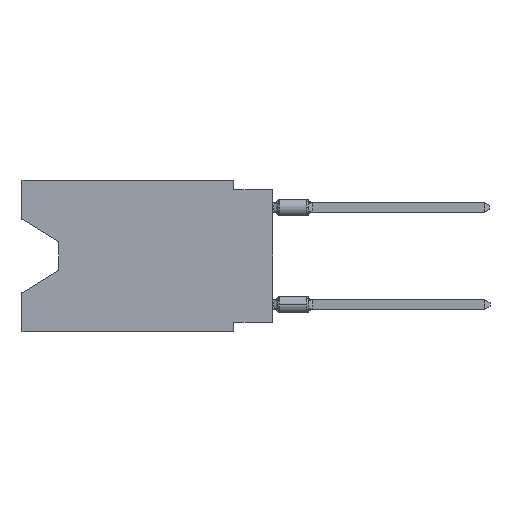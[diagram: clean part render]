
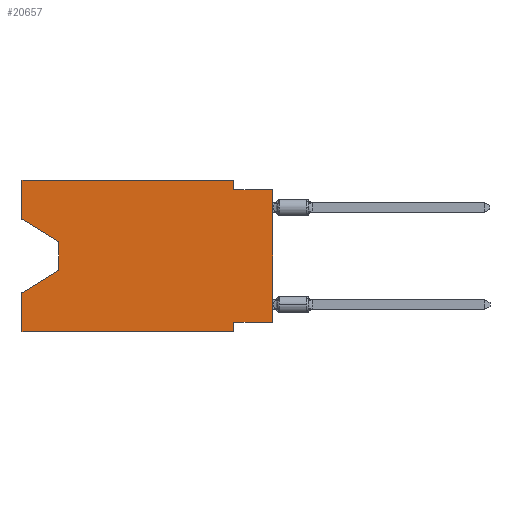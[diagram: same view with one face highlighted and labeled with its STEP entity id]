
A CAD part, left-side view. The second image highlights one B-rep face of the part: STEP entity #20657.
In plain terms, the highlighted planar face has unit normal (-1, 0, 0).
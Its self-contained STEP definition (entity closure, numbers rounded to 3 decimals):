
#172 = CARTESIAN_POINT ( 'NONE',  ( 0., 13.97, -4.013 ) ) ;
#270 = CARTESIAN_POINT ( 'NONE',  ( 0., 16.383, 0. ) ) ;
#666 = CARTESIAN_POINT ( 'NONE',  ( 0., 0., -0.635 ) ) ;
#1020 = CARTESIAN_POINT ( 'NONE',  ( 0., 13.97, -5.893 ) ) ;
#1090 = VERTEX_POINT ( 'NONE', #17927 ) ;
#1123 = ORIENTED_EDGE ( 'NONE', *, *, #8444, .T. ) ;
#1266 = VECTOR ( 'NONE', #6108, 1000. ) ;
#1345 = EDGE_CURVE ( 'NONE', #3712, #14946, #4710, .T. ) ;
#1466 = DIRECTION ( 'NONE',  ( 0., 0., 1. ) ) ;
#2115 = LINE ( 'NONE', #22886, #17380 ) ;
#2216 = PLANE ( 'NONE',  #22146 ) ;
#2451 = DIRECTION ( 'NONE',  ( 1., 0., 0. ) ) ;
#2823 = DIRECTION ( 'NONE',  ( 0., -1., 0. ) ) ;
#3032 = EDGE_CURVE ( 'NONE', #1090, #3712, #23635, .T. ) ;
#3294 = CARTESIAN_POINT ( 'NONE',  ( 0., 0., 0. ) ) ;
#3623 = VECTOR ( 'NONE', #15454, 1000. ) ;
#3646 = DIRECTION ( 'NONE',  ( 0., -1., 0. ) ) ;
#3660 = VECTOR ( 'NONE', #1466, 1000. ) ;
#3712 = VERTEX_POINT ( 'NONE', #14829 ) ;
#3999 = EDGE_CURVE ( 'NONE', #6644, #1090, #4670, .T. ) ;
#4010 = CARTESIAN_POINT ( 'NONE',  ( 0., 16.383, -2.546 ) ) ;
#4031 = CARTESIAN_POINT ( 'NONE',  ( 0., 16.383, -2.546 ) ) ;
#4294 = VERTEX_POINT ( 'NONE', #12176 ) ;
#4529 = VERTEX_POINT ( 'NONE', #20146 ) ;
#4670 = LINE ( 'NONE', #4904, #5822 ) ;
#4710 = LINE ( 'NONE', #666, #17588 ) ;
#4880 = ORIENTED_EDGE ( 'NONE', *, *, #17464, .F. ) ;
#4904 = CARTESIAN_POINT ( 'NONE',  ( 0., 16.383, 0. ) ) ;
#5822 = VECTOR ( 'NONE', #2823, 1000. ) ;
#5956 = VECTOR ( 'NONE', #19728, 1000. ) ;
#6108 = DIRECTION ( 'NONE',  ( 0., 0., -1. ) ) ;
#6146 = DIRECTION ( 'NONE',  ( 0., 0., -1. ) ) ;
#6256 = ORIENTED_EDGE ( 'NONE', *, *, #12687, .T. ) ;
#6288 = VERTEX_POINT ( 'NONE', #1020 ) ;
#6576 = DIRECTION ( 'NONE',  ( 0., 1., 0. ) ) ;
#6644 = VERTEX_POINT ( 'NONE', #270 ) ;
#6875 = CARTESIAN_POINT ( 'NONE',  ( 0., 2.54, 0. ) ) ;
#7000 = ORIENTED_EDGE ( 'NONE', *, *, #1345, .F. ) ;
#7571 = LINE ( 'NONE', #14782, #22473 ) ;
#7693 = CARTESIAN_POINT ( 'NONE',  ( 0., 16.383, -9.906 ) ) ;
#7701 = ORIENTED_EDGE ( 'NONE', *, *, #3032, .F. ) ;
#8292 = CARTESIAN_POINT ( 'NONE',  ( 0., 0., -9.271 ) ) ;
#8444 = EDGE_CURVE ( 'NONE', #23973, #6288, #2115, .T. ) ;
#8842 = CARTESIAN_POINT ( 'NONE',  ( 0., 16.383, 0. ) ) ;
#9083 = VERTEX_POINT ( 'NONE', #11960 ) ;
#9902 = DIRECTION ( 'NONE',  ( 0., 0., -1. ) ) ;
#10111 = LINE ( 'NONE', #8292, #21244 ) ;
#10466 = VERTEX_POINT ( 'NONE', #4010 ) ;
#10877 = ORIENTED_EDGE ( 'NONE', *, *, #16063, .T. ) ;
#10914 = VERTEX_POINT ( 'NONE', #22311 ) ;
#11291 = CARTESIAN_POINT ( 'NONE',  ( 0., 16.383, -7.36 ) ) ;
#11810 = DIRECTION ( 'NONE',  ( 0., -1., 0. ) ) ;
#11960 = CARTESIAN_POINT ( 'NONE',  ( 0., 2.54, -9.906 ) ) ;
#12037 = ORIENTED_EDGE ( 'NONE', *, *, #16040, .T. ) ;
#12176 = CARTESIAN_POINT ( 'NONE',  ( 0., 16.383, -9.906 ) ) ;
#12626 = DIRECTION ( 'NONE',  ( 0., 0., 1. ) ) ;
#12687 = EDGE_CURVE ( 'NONE', #10466, #23973, #19079, .T. ) ;
#12725 = EDGE_CURVE ( 'NONE', #10914, #9083, #22850, .T. ) ;
#12735 = VECTOR ( 'NONE', #3646, 1000. ) ;
#12946 = ORIENTED_EDGE ( 'NONE', *, *, #23197, .F. ) ;
#13121 = EDGE_CURVE ( 'NONE', #10466, #6644, #19500, .T. ) ;
#13352 = FACE_OUTER_BOUND ( 'NONE', #23119, .T. ) ;
#13728 = EDGE_CURVE ( 'NONE', #4529, #14946, #14438, .T. ) ;
#14003 = ORIENTED_EDGE ( 'NONE', *, *, #3999, .F. ) ;
#14318 = ORIENTED_EDGE ( 'NONE', *, *, #13121, .F. ) ;
#14438 = LINE ( 'NONE', #3294, #3660 ) ;
#14782 = CARTESIAN_POINT ( 'NONE',  ( 0., 13.97, -5.893 ) ) ;
#14829 = CARTESIAN_POINT ( 'NONE',  ( 0., 2.54, -0.635 ) ) ;
#14946 = VERTEX_POINT ( 'NONE', #17848 ) ;
#15454 = DIRECTION ( 'NONE',  ( 0., 0., 1. ) ) ;
#15495 = VECTOR ( 'NONE', #12626, 1000. ) ;
#15569 = CARTESIAN_POINT ( 'NONE',  ( 0., 16.383, 0. ) ) ;
#16040 = EDGE_CURVE ( 'NONE', #6288, #20054, #7571, .T. ) ;
#16063 = EDGE_CURVE ( 'NONE', #4294, #9083, #22114, .T. ) ;
#17380 = VECTOR ( 'NONE', #6146, 1000. ) ;
#17464 = EDGE_CURVE ( 'NONE', #4529, #10914, #10111, .T. ) ;
#17572 = ORIENTED_EDGE ( 'NONE', *, *, #12725, .F. ) ;
#17588 = VECTOR ( 'NONE', #11810, 1000. ) ;
#17848 = CARTESIAN_POINT ( 'NONE',  ( 0., 0., -0.635 ) ) ;
#17927 = CARTESIAN_POINT ( 'NONE',  ( 0., 2.54, 0. ) ) ;
#18877 = VECTOR ( 'NONE', #18957, 1000. ) ;
#18957 = DIRECTION ( 'NONE',  ( 0., -0.855, -0.519 ) ) ;
#19079 = LINE ( 'NONE', #4031, #18877 ) ;
#19500 = LINE ( 'NONE', #15569, #3623 ) ;
#19728 = DIRECTION ( 'NONE',  ( 0., 0., -1. ) ) ;
#20054 = VERTEX_POINT ( 'NONE', #11291 ) ;
#20146 = CARTESIAN_POINT ( 'NONE',  ( 0., 0., -9.271 ) ) ;
#20282 = DIRECTION ( 'NONE',  ( 0., 0.855, -0.519 ) ) ;
#20325 = LINE ( 'NONE', #8842, #15495 ) ;
#20459 = ORIENTED_EDGE ( 'NONE', *, *, #13728, .T. ) ;
#20657 = ADVANCED_FACE ( 'NONE', ( #13352 ), #2216, .F. ) ;
#21244 = VECTOR ( 'NONE', #6576, 1000. ) ;
#22114 = LINE ( 'NONE', #7693, #12735 ) ;
#22146 = AXIS2_PLACEMENT_3D ( 'NONE', #22871, #2451, #9902 ) ;
#22311 = CARTESIAN_POINT ( 'NONE',  ( 0., 2.54, -9.271 ) ) ;
#22473 = VECTOR ( 'NONE', #20282, 1000. ) ;
#22616 = CARTESIAN_POINT ( 'NONE',  ( 0., 2.54, -9.906 ) ) ;
#22850 = LINE ( 'NONE', #22616, #1266 ) ;
#22871 = CARTESIAN_POINT ( 'NONE',  ( 0., 16.383, 0. ) ) ;
#22886 = CARTESIAN_POINT ( 'NONE',  ( 0., 13.97, -4.013 ) ) ;
#23119 = EDGE_LOOP ( 'NONE', ( #6256, #1123, #12037, #12946, #10877, #17572, #4880, #20459, #7000, #7701, #14003, #14318 ) ) ;
#23197 = EDGE_CURVE ( 'NONE', #4294, #20054, #20325, .T. ) ;
#23635 = LINE ( 'NONE', #6875, #5956 ) ;
#23973 = VERTEX_POINT ( 'NONE', #172 ) ;
